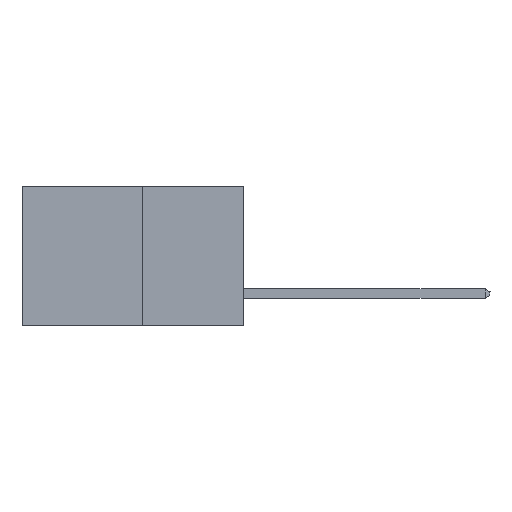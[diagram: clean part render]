
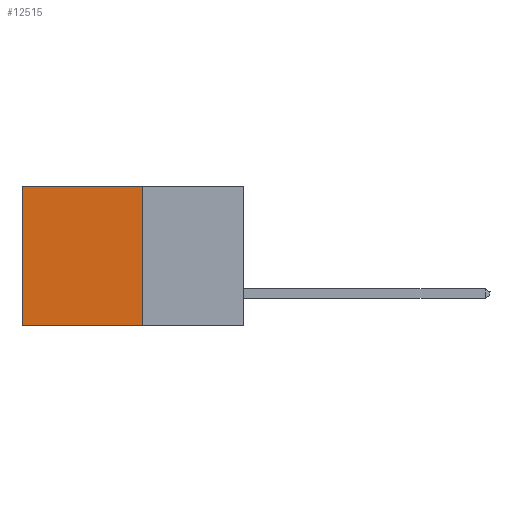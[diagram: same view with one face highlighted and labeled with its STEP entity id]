
A CAD part, left-side view. The second image highlights one B-rep face of the part: STEP entity #12515.
In plain terms, the highlighted planar face has unit normal (-1, 0, 0).
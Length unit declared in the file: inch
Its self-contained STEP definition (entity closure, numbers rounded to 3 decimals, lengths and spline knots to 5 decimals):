
#1472 = LINE ( 'NONE', #5578, #9149 ) ;
#1597 = LINE ( 'NONE', #11222, #5864 ) ;
#1696 = VERTEX_POINT ( 'NONE', #16330 ) ;
#2104 = CARTESIAN_POINT ( 'NONE',  ( 0.277, 0.59, 0. ) ) ;
#2572 = DIRECTION ( 'NONE',  ( 0., 0., -1. ) ) ;
#2705 = VECTOR ( 'NONE', #5610, 39.37008 ) ;
#2764 = ORIENTED_EDGE ( 'NONE', *, *, #7521, .T. ) ;
#2809 = DIRECTION ( 'NONE',  ( 0., 1., 0. ) ) ;
#2930 = VERTEX_POINT ( 'NONE', #9561 ) ;
#3259 = VERTEX_POINT ( 'NONE', #2104 ) ;
#4269 = EDGE_CURVE ( 'NONE', #2930, #1696, #1472, .T. ) ;
#4971 = LINE ( 'NONE', #11453, #9277 ) ;
#5578 = CARTESIAN_POINT ( 'NONE',  ( 0.277, 0.27, -0.37 ) ) ;
#5610 = DIRECTION ( 'NONE',  ( 0., 1., 0. ) ) ;
#5864 = VECTOR ( 'NONE', #6921, 39.37008 ) ;
#6921 = DIRECTION ( 'NONE',  ( 0., 0., -1. ) ) ;
#7521 = EDGE_CURVE ( 'NONE', #3259, #18274, #1597, .T. ) ;
#8794 = EDGE_CURVE ( 'NONE', #2930, #3259, #17473, .T. ) ;
#9149 = VECTOR ( 'NONE', #9893, 39.37008 ) ;
#9277 = VECTOR ( 'NONE', #2809, 39.37008 ) ;
#9561 = CARTESIAN_POINT ( 'NONE',  ( 0.277, 0.27, 0. ) ) ;
#9768 = CARTESIAN_POINT ( 'NONE',  ( 0.277, 0.27, -0.37 ) ) ;
#9893 = DIRECTION ( 'NONE',  ( 0., 0., -1. ) ) ;
#9974 = ORIENTED_EDGE ( 'NONE', *, *, #14526, .F. ) ;
#10487 = FACE_OUTER_BOUND ( 'NONE', #13835, .T. ) ;
#11213 = DIRECTION ( 'NONE',  ( 1., 0., 0. ) ) ;
#11222 = CARTESIAN_POINT ( 'NONE',  ( 0.277, 0.59, -0.37 ) ) ;
#11453 = CARTESIAN_POINT ( 'NONE',  ( 0.277, 0.27, -0.37 ) ) ;
#12515 = ADVANCED_FACE ( 'NONE', ( #10487 ), #18252, .F. ) ;
#13835 = EDGE_LOOP ( 'NONE', ( #2764, #9974, #17335, #17834 ) ) ;
#14526 = EDGE_CURVE ( 'NONE', #1696, #18274, #4971, .T. ) ;
#14620 = CARTESIAN_POINT ( 'NONE',  ( 0.277, 0.59, -0.37 ) ) ;
#16330 = CARTESIAN_POINT ( 'NONE',  ( 0.277, 0.27, -0.37 ) ) ;
#16686 = AXIS2_PLACEMENT_3D ( 'NONE', #9768, #11213, #2572 ) ;
#17335 = ORIENTED_EDGE ( 'NONE', *, *, #4269, .F. ) ;
#17473 = LINE ( 'NONE', #18451, #2705 ) ;
#17834 = ORIENTED_EDGE ( 'NONE', *, *, #8794, .T. ) ;
#18252 = PLANE ( 'NONE',  #16686 ) ;
#18274 = VERTEX_POINT ( 'NONE', #14620 ) ;
#18451 = CARTESIAN_POINT ( 'NONE',  ( 0.277, 0.27, 0. ) ) ;
